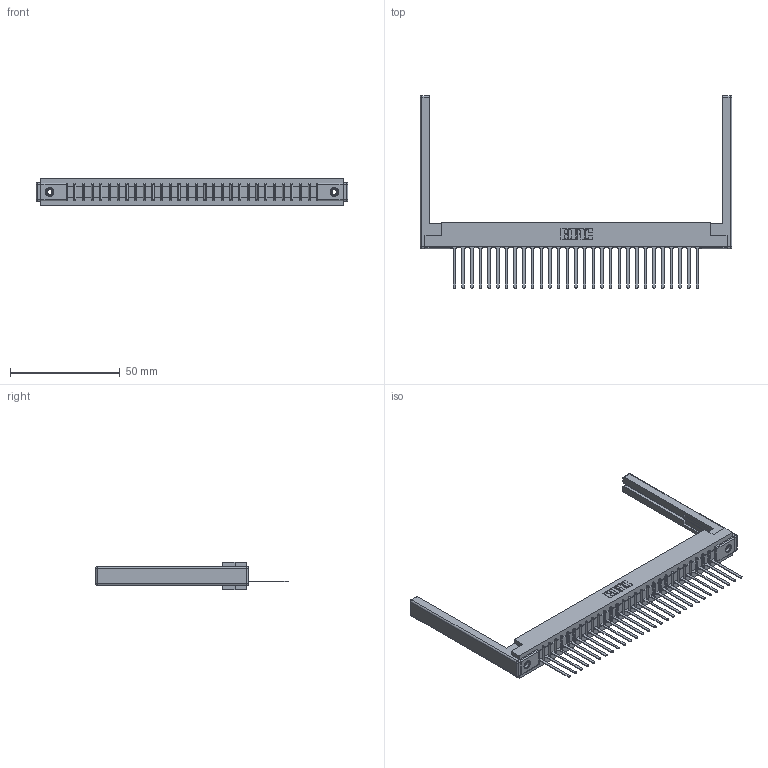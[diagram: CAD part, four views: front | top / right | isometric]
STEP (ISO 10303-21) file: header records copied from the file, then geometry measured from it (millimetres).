
FILE_DESCRIPTION (( 'STEP AP203' ), '1' );
FILE_NAME ('357-029-545-168.STEP', '2019-09-14T03:42:51', ( '' ), ( '' ), 'SwSTEP 2.0', 'SolidWorks 2016', '' );
FILE_SCHEMA (( 'CONFIG_CONTROL_DESIGN' ));
Length unit declared in the file: inch
Products named in the file (5): 357-029-545-168; 345-250-001_345-250-001-102; 307 Part_.156 Dia Mounting Holes; 307-220-068; 307-290-001_545
Assembly tree (34 placements, depth 2):
  357-029-545-168
    307 Part_.156 Dia Mounting Holes
    307-290-001_545  x29
    307-220-068  x2
    345-250-001_345-250-001-102  x2
Bounding box: 142.34 x 87.96 x 12.7 mm (x, y, z)
Volume: 19212.6 mm3; surface area: 20378.4 mm2
Topology: 34 solids, 34 shells, 1926 faces, 5411 edges, 3466 vertices
Faces by surface type: plane 1231, cylinder 611, sphere 68, cone 12, torus 4
Entity records: 29191 total; most frequent: CARTESIAN_POINT 4877, ORIENTED_EDGE 4852, DIRECTION 4768, EDGE_CURVE 2426, VECTOR 1854, LINE 1854, VERTEX_POINT 1566, AXIS2_PLACEMENT_3D 1457
